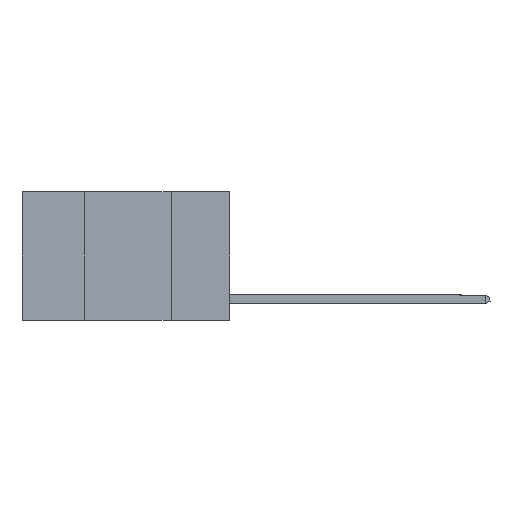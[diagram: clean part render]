
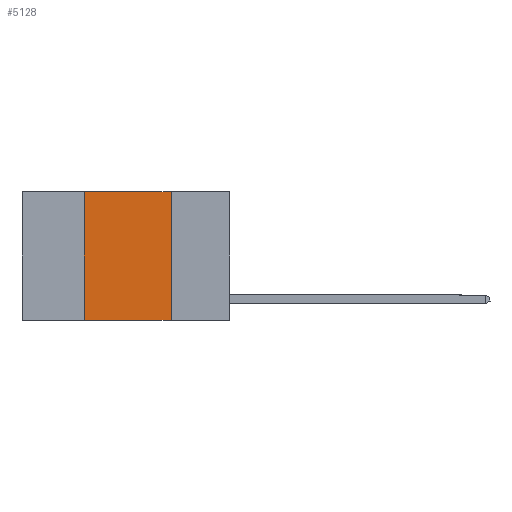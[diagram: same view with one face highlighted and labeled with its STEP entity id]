
A CAD part, left-side view. The second image highlights one B-rep face of the part: STEP entity #5128.
In plain terms, the highlighted planar face has unit normal (-1, 0, 0).
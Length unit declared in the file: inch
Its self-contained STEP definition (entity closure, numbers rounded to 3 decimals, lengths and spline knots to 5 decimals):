
#172 = EDGE_CURVE ( 'NONE', #9478, #7394, #12998, .T. ) ;
#903 = CARTESIAN_POINT ( 'NONE',  ( 0., 0.17, -0.37 ) ) ;
#1101 = EDGE_CURVE ( 'NONE', #7394, #10184, #6339, .T. ) ;
#1380 = DIRECTION ( 'NONE',  ( 0., -1., 0. ) ) ;
#1392 = CARTESIAN_POINT ( 'NONE',  ( 0., 0.42, -0.37 ) ) ;
#1846 = LINE ( 'NONE', #10785, #4292 ) ;
#3235 = DIRECTION ( 'NONE',  ( 0., 0., 1. ) ) ;
#3343 = ORIENTED_EDGE ( 'NONE', *, *, #172, .F. ) ;
#4162 = FACE_OUTER_BOUND ( 'NONE', #10060, .T. ) ;
#4292 = VECTOR ( 'NONE', #1380, 39.37008 ) ;
#5128 = ADVANCED_FACE ( 'NONE', ( #4162 ), #5299, .F. ) ;
#5299 = PLANE ( 'NONE',  #11624 ) ;
#5351 = DIRECTION ( 'NONE',  ( 0., 0., -1. ) ) ;
#6142 = CARTESIAN_POINT ( 'NONE',  ( 0., 0.42, 0. ) ) ;
#6321 = DIRECTION ( 'NONE',  ( 1., 0., 0. ) ) ;
#6339 = LINE ( 'NONE', #8042, #8825 ) ;
#6355 = VERTEX_POINT ( 'NONE', #903 ) ;
#6368 = DIRECTION ( 'NONE',  ( 0., 0., -1. ) ) ;
#6392 = CARTESIAN_POINT ( 'NONE',  ( 0., 0.42, 0. ) ) ;
#6636 = EDGE_CURVE ( 'NONE', #9478, #6355, #1846, .T. ) ;
#7394 = VERTEX_POINT ( 'NONE', #6392 ) ;
#8042 = CARTESIAN_POINT ( 'NONE',  ( 0., 0.6, 0. ) ) ;
#8643 = ORIENTED_EDGE ( 'NONE', *, *, #1101, .F. ) ;
#8671 = ORIENTED_EDGE ( 'NONE', *, *, #6636, .T. ) ;
#8825 = VECTOR ( 'NONE', #8990, 39.37008 ) ;
#8990 = DIRECTION ( 'NONE',  ( 0., -1., 0. ) ) ;
#9478 = VERTEX_POINT ( 'NONE', #1392 ) ;
#9943 = EDGE_CURVE ( 'NONE', #10184, #6355, #12417, .T. ) ;
#10060 = EDGE_LOOP ( 'NONE', ( #10391, #8643, #3343, #8671 ) ) ;
#10184 = VERTEX_POINT ( 'NONE', #10906 ) ;
#10269 = VECTOR ( 'NONE', #3235, 39.37008 ) ;
#10391 = ORIENTED_EDGE ( 'NONE', *, *, #9943, .F. ) ;
#10498 = CARTESIAN_POINT ( 'NONE',  ( 0., 0.6, 0. ) ) ;
#10785 = CARTESIAN_POINT ( 'NONE',  ( 0., 0.6, -0.37 ) ) ;
#10906 = CARTESIAN_POINT ( 'NONE',  ( 0., 0.17, 0. ) ) ;
#11579 = CARTESIAN_POINT ( 'NONE',  ( 0., 0.17, 0. ) ) ;
#11624 = AXIS2_PLACEMENT_3D ( 'NONE', #10498, #6321, #6368 ) ;
#12417 = LINE ( 'NONE', #11579, #12750 ) ;
#12750 = VECTOR ( 'NONE', #5351, 39.37008 ) ;
#12998 = LINE ( 'NONE', #6142, #10269 ) ;
